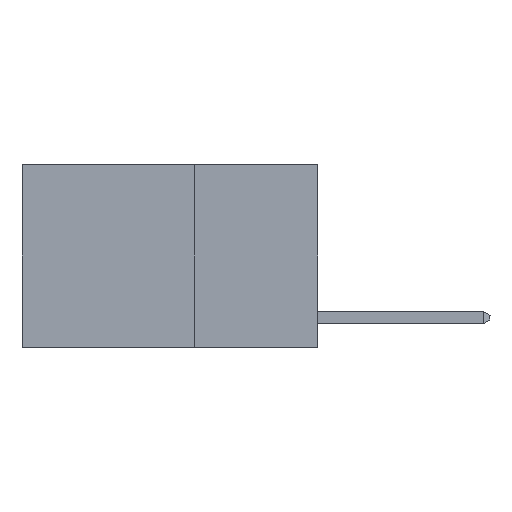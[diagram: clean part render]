
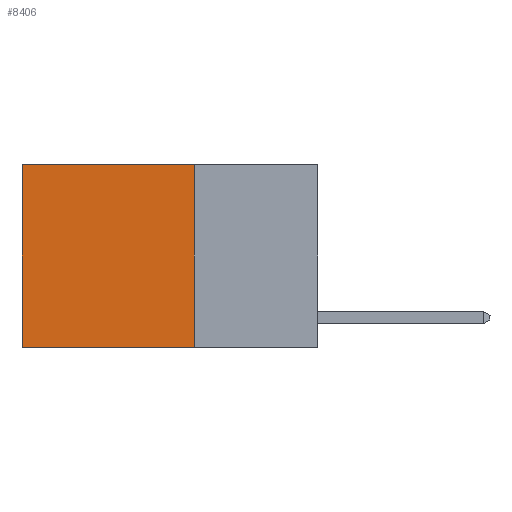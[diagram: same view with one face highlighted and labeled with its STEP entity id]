
A CAD part, left-side view. The second image highlights one B-rep face of the part: STEP entity #8406.
In plain terms, the highlighted planar face has unit normal (-1, 0, 0).
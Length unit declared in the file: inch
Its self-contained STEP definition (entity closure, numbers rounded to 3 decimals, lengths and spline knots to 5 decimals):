
#363 = CARTESIAN_POINT ( 'NONE',  ( 0.2625, 0.25, -0.37 ) ) ;
#1052 = EDGE_CURVE ( 'NONE', #3349, #11822, #9460, .T. ) ;
#1932 = VERTEX_POINT ( 'NONE', #12696 ) ;
#2019 = CARTESIAN_POINT ( 'NONE',  ( 0.2625, 0.25, 0. ) ) ;
#2589 = CARTESIAN_POINT ( 'NONE',  ( 0.2625, 0.6, -0.37 ) ) ;
#3181 = CARTESIAN_POINT ( 'NONE',  ( 0.2625, 0.6, 0. ) ) ;
#3245 = VECTOR ( 'NONE', #7388, 39.37008 ) ;
#3297 = ORIENTED_EDGE ( 'NONE', *, *, #8660, .T. ) ;
#3349 = VERTEX_POINT ( 'NONE', #363 ) ;
#5445 = AXIS2_PLACEMENT_3D ( 'NONE', #7445, #14725, #7554 ) ;
#5482 = VECTOR ( 'NONE', #15255, 39.37008 ) ;
#5533 = DIRECTION ( 'NONE',  ( 0., 1., 0. ) ) ;
#5778 = CARTESIAN_POINT ( 'NONE',  ( 0.2625, 0.25, 0. ) ) ;
#7082 = CARTESIAN_POINT ( 'NONE',  ( 0.2625, 0.25, 0. ) ) ;
#7388 = DIRECTION ( 'NONE',  ( 0., 1., 0. ) ) ;
#7445 = CARTESIAN_POINT ( 'NONE',  ( 0.2625, 0.25, 0. ) ) ;
#7554 = DIRECTION ( 'NONE',  ( 0., 0., -1. ) ) ;
#7979 = ORIENTED_EDGE ( 'NONE', *, *, #8142, .F. ) ;
#7984 = FACE_OUTER_BOUND ( 'NONE', #8184, .T. ) ;
#7989 = ORIENTED_EDGE ( 'NONE', *, *, #9994, .T. ) ;
#8142 = EDGE_CURVE ( 'NONE', #15227, #3349, #15270, .T. ) ;
#8184 = EDGE_LOOP ( 'NONE', ( #3297, #14091, #7979, #7989 ) ) ;
#8372 = VECTOR ( 'NONE', #10615, 39.37008 ) ;
#8406 = ADVANCED_FACE ( 'NONE', ( #7984 ), #13657, .F. ) ;
#8660 = EDGE_CURVE ( 'NONE', #1932, #11822, #9121, .T. ) ;
#9121 = LINE ( 'NONE', #3181, #5482 ) ;
#9460 = LINE ( 'NONE', #15377, #11553 ) ;
#9994 = EDGE_CURVE ( 'NONE', #15227, #1932, #11707, .T. ) ;
#10615 = DIRECTION ( 'NONE',  ( 0., 0., -1. ) ) ;
#11553 = VECTOR ( 'NONE', #5533, 39.37008 ) ;
#11707 = LINE ( 'NONE', #7082, #3245 ) ;
#11822 = VERTEX_POINT ( 'NONE', #2589 ) ;
#12696 = CARTESIAN_POINT ( 'NONE',  ( 0.2625, 0.6, 0. ) ) ;
#13657 = PLANE ( 'NONE',  #5445 ) ;
#14091 = ORIENTED_EDGE ( 'NONE', *, *, #1052, .F. ) ;
#14725 = DIRECTION ( 'NONE',  ( 1., 0., 0. ) ) ;
#15227 = VERTEX_POINT ( 'NONE', #5778 ) ;
#15255 = DIRECTION ( 'NONE',  ( 0., 0., -1. ) ) ;
#15270 = LINE ( 'NONE', #2019, #8372 ) ;
#15377 = CARTESIAN_POINT ( 'NONE',  ( 0.2625, 0.25, -0.37 ) ) ;
